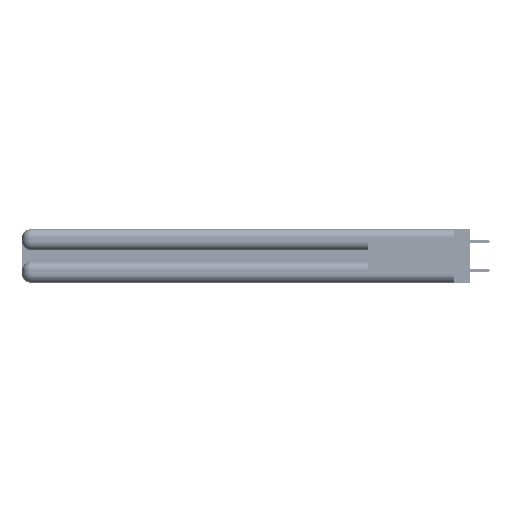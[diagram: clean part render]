
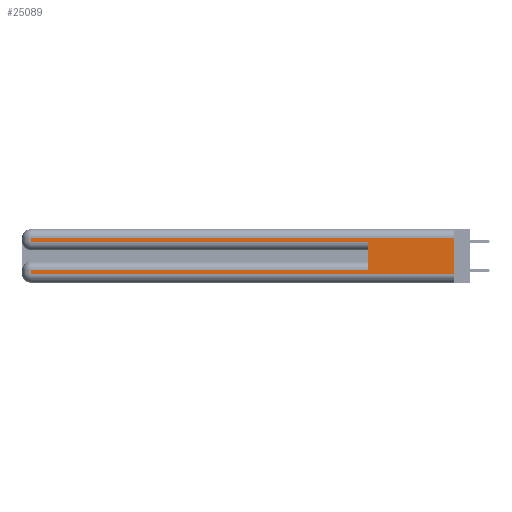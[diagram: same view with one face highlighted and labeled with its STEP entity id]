
A CAD part, left-side view. The second image highlights one B-rep face of the part: STEP entity #25089.
In plain terms, the highlighted planar face has unit normal (-1, 0, 0).
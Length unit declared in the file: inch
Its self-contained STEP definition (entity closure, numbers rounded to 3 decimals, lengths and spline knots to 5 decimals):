
#736 = CARTESIAN_POINT ( 'NONE',  ( 0., 0., 0.285 ) ) ;
#1190 = DIRECTION ( 'NONE',  ( 0., 0., -1. ) ) ;
#2565 = EDGE_CURVE ( 'NONE', #32001, #49664, #39038, .T. ) ;
#3140 = ORIENTED_EDGE ( 'NONE', *, *, #48642, .F. ) ;
#4144 = VERTEX_POINT ( 'NONE', #20246 ) ;
#5531 = EDGE_CURVE ( 'NONE', #44752, #19418, #12230, .T. ) ;
#5854 = CARTESIAN_POINT ( 'NONE',  ( 0., 2.94, 0.37 ) ) ;
#9098 = CARTESIAN_POINT ( 'NONE',  ( 0., 0., 0.085 ) ) ;
#9511 = DIRECTION ( 'NONE',  ( 1., 0., 0. ) ) ;
#10490 = EDGE_CURVE ( 'NONE', #20601, #4144, #51126, .T. ) ;
#11422 = LINE ( 'NONE', #32408, #29004 ) ;
#12230 = LINE ( 'NONE', #29071, #53311 ) ;
#13468 = CARTESIAN_POINT ( 'NONE',  ( 0., 2.94, 0.06 ) ) ;
#14210 = FACE_OUTER_BOUND ( 'NONE', #49649, .T. ) ;
#17195 = CARTESIAN_POINT ( 'NONE',  ( 0., 0.6, 0.085 ) ) ;
#17624 = VERTEX_POINT ( 'NONE', #24758 ) ;
#17959 = DIRECTION ( 'NONE',  ( 0., 1., 0. ) ) ;
#19418 = VERTEX_POINT ( 'NONE', #27570 ) ;
#19523 = CARTESIAN_POINT ( 'NONE',  ( 0., 2.94, 0.37 ) ) ;
#19613 = CARTESIAN_POINT ( 'NONE',  ( 0., 0., 0.37 ) ) ;
#19795 = DIRECTION ( 'NONE',  ( 0., 0., -1. ) ) ;
#20246 = CARTESIAN_POINT ( 'NONE',  ( 0., 2.94, 0.085 ) ) ;
#20601 = VERTEX_POINT ( 'NONE', #17195 ) ;
#22507 = CARTESIAN_POINT ( 'NONE',  ( 0., 0., 0.37 ) ) ;
#24201 = AXIS2_PLACEMENT_3D ( 'NONE', #22507, #9511, #1190 ) ;
#24758 = CARTESIAN_POINT ( 'NONE',  ( 0., 0.6, 0.285 ) ) ;
#25089 = ADVANCED_FACE ( 'NONE', ( #14210 ), #31050, .F. ) ;
#27570 = CARTESIAN_POINT ( 'NONE',  ( 0., 0., 0.06 ) ) ;
#27613 = LINE ( 'NONE', #19613, #32251 ) ;
#28620 = LINE ( 'NONE', #19523, #34366 ) ;
#29004 = VECTOR ( 'NONE', #37103, 39.37008 ) ;
#29071 = CARTESIAN_POINT ( 'NONE',  ( 0., 0., 0.06 ) ) ;
#30045 = DIRECTION ( 'NONE',  ( 0., -1., 0. ) ) ;
#31050 = PLANE ( 'NONE',  #24201 ) ;
#32001 = VERTEX_POINT ( 'NONE', #34387 ) ;
#32251 = VECTOR ( 'NONE', #44477, 39.37008 ) ;
#32312 = EDGE_CURVE ( 'NONE', #53064, #32001, #11422, .T. ) ;
#32408 = CARTESIAN_POINT ( 'NONE',  ( 0., 0., 0.31 ) ) ;
#32910 = ORIENTED_EDGE ( 'NONE', *, *, #2565, .T. ) ;
#33078 = CARTESIAN_POINT ( 'NONE',  ( 0., 0.6, 0.145 ) ) ;
#33169 = CARTESIAN_POINT ( 'NONE',  ( 0., 0., 0.31 ) ) ;
#33213 = EDGE_CURVE ( 'NONE', #4144, #44752, #28620, .T. ) ;
#34366 = VECTOR ( 'NONE', #19795, 39.37008 ) ;
#34387 = CARTESIAN_POINT ( 'NONE',  ( 0., 2.94, 0.31 ) ) ;
#35027 = ORIENTED_EDGE ( 'NONE', *, *, #47765, .F. ) ;
#35162 = DIRECTION ( 'NONE',  ( 0., 0., -1. ) ) ;
#37103 = DIRECTION ( 'NONE',  ( 0., 1., 0. ) ) ;
#37984 = ORIENTED_EDGE ( 'NONE', *, *, #33213, .T. ) ;
#39038 = LINE ( 'NONE', #5854, #43869 ) ;
#41119 = CARTESIAN_POINT ( 'NONE',  ( 0., 2.94, 0.285 ) ) ;
#41466 = EDGE_CURVE ( 'NONE', #49664, #17624, #42496, .T. ) ;
#41663 = DIRECTION ( 'NONE',  ( 0., 0., 1. ) ) ;
#41767 = ORIENTED_EDGE ( 'NONE', *, *, #41466, .T. ) ;
#42332 = DIRECTION ( 'NONE',  ( 0., -1., 0. ) ) ;
#42496 = LINE ( 'NONE', #736, #44191 ) ;
#43338 = ORIENTED_EDGE ( 'NONE', *, *, #32312, .T. ) ;
#43869 = VECTOR ( 'NONE', #35162, 39.37008 ) ;
#44191 = VECTOR ( 'NONE', #30045, 39.37008 ) ;
#44477 = DIRECTION ( 'NONE',  ( 0., 0., -1. ) ) ;
#44568 = VECTOR ( 'NONE', #41663, 39.37008 ) ;
#44670 = VECTOR ( 'NONE', #17959, 39.37008 ) ;
#44752 = VERTEX_POINT ( 'NONE', #13468 ) ;
#46719 = ORIENTED_EDGE ( 'NONE', *, *, #5531, .T. ) ;
#47257 = ORIENTED_EDGE ( 'NONE', *, *, #10490, .T. ) ;
#47765 = EDGE_CURVE ( 'NONE', #53064, #19418, #27613, .T. ) ;
#48642 = EDGE_CURVE ( 'NONE', #20601, #17624, #50242, .T. ) ;
#49649 = EDGE_LOOP ( 'NONE', ( #35027, #43338, #32910, #41767, #3140, #47257, #37984, #46719 ) ) ;
#49664 = VERTEX_POINT ( 'NONE', #41119 ) ;
#50242 = LINE ( 'NONE', #33078, #44568 ) ;
#51126 = LINE ( 'NONE', #9098, #44670 ) ;
#53064 = VERTEX_POINT ( 'NONE', #33169 ) ;
#53311 = VECTOR ( 'NONE', #42332, 39.37008 ) ;
